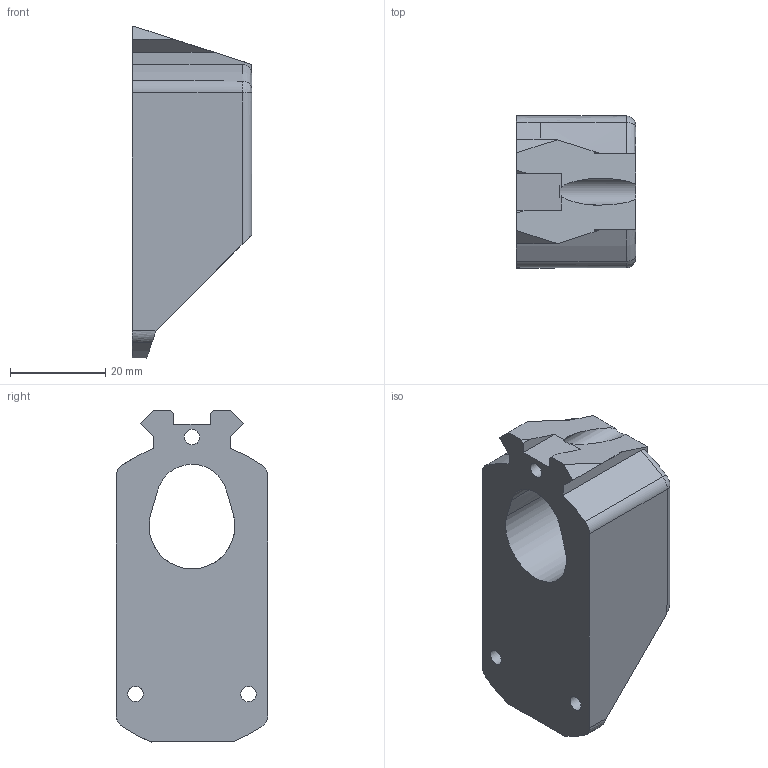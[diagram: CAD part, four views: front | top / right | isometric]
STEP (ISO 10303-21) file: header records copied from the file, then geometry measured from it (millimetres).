
FILE_DESCRIPTION(/* description */ (''),/* implementation_level */ '2;1');
FILE_NAME(/* name */ 'end cap.step',/* time_stamp */ '2021-09-02T19:31:22-05:00',/* author */ (''),/* organization */ (''),/* preprocessor_version */ 'ST-DEVELOPER v18.1',/* originating_system */ 'Autodesk Translation Framework v10.10.0.1391',/* authorisation */ '');
FILE_SCHEMA (('AUTOMOTIVE_DESIGN { 1 0 10303 214 3 1 1 }'));
Length unit declared in the file: millimetre
Products named in the file (1): end cap
Bounding box: 25.11 x 31.81 x 69.62 mm (x, y, z)
Volume: 30883.4 mm3; surface area: 9014.9 mm2
Topology: 1 solids, 1 shells, 132 faces, 365 edges, 241 vertices
Faces by surface type: bspline 87, plane 36, cylinder 9
Full cylindrical faces by diameter (mm): 3.25 x3, 5.65 x2
Entity records: 4806 total; most frequent: CARTESIAN_POINT 2181, ORIENTED_EDGE 730, EDGE_CURVE 365, DIRECTION 304, VERTEX_POINT 241, LINE 164, VECTOR 164, EDGE_LOOP 146
